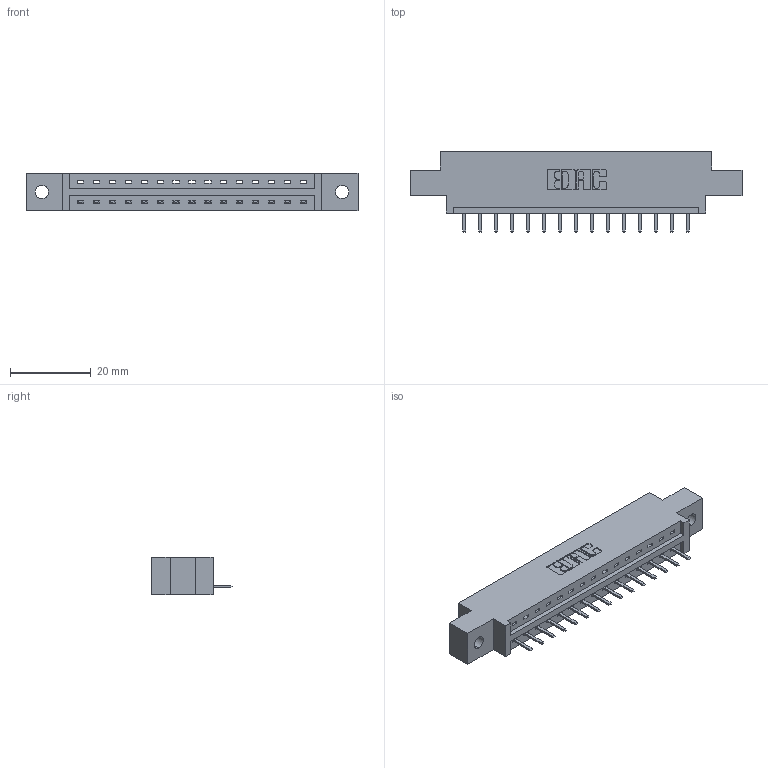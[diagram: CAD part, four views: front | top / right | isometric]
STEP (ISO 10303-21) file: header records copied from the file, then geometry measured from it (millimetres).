
FILE_DESCRIPTION (( 'STEP AP203' ), '1' );
FILE_NAME ('337-015-520-602.STEP', '2019-09-28T16:18:28', ( '' ), ( '' ), 'SwSTEP 2.0', 'SolidWorks 2016', '' );
FILE_SCHEMA (( 'CONFIG_CONTROL_DESIGN' ));
Length unit declared in the file: inch
Products named in the file (3): 345-292-001_345-293-120; 337-015-520-602; 337 Part_0.170 Offset - 0.128 Dia
Assembly tree (16 placements, depth 2):
  337-015-520-602
    337 Part_0.170 Offset - 0.128 Dia
    345-292-001_345-293-120  x15
Bounding box: 82.45 x 20.02 x 9.4 mm (x, y, z)
Volume: 8033.9 mm3; surface area: 7823.3 mm2
Topology: 16 solids, 16 shells, 1108 faces, 3263 edges, 2134 vertices
Faces by surface type: plane 794, cylinder 314
Entity records: 14891 total; most frequent: CARTESIAN_POINT 2611, ORIENTED_EDGE 2550, DIRECTION 2241, EDGE_CURVE 1275, VECTOR 1143, LINE 1143, VERTEX_POINT 846, AXIS2_PLACEMENT_3D 549
